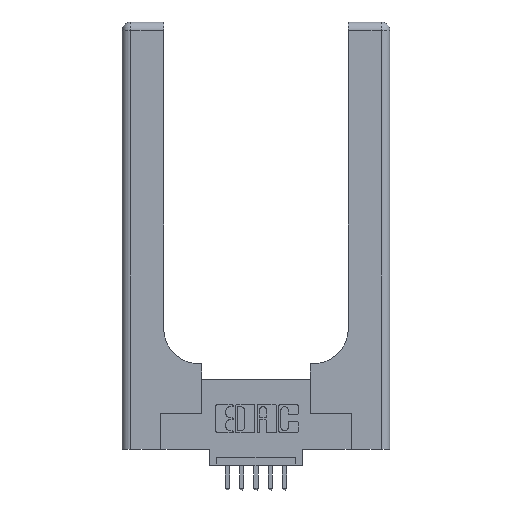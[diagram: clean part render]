
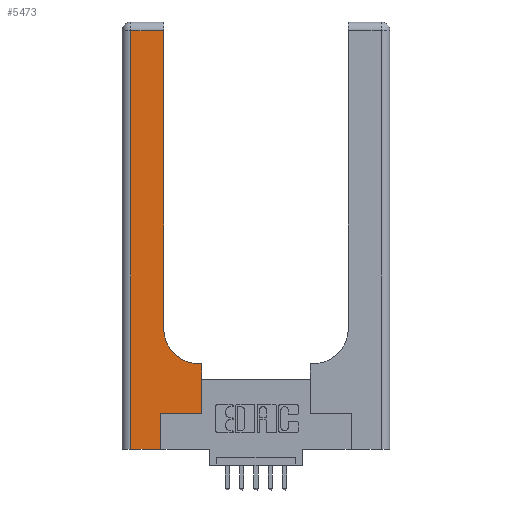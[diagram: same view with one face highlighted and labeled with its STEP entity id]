
A CAD part, top view. The second image highlights one B-rep face of the part: STEP entity #5473.
In plain terms, the highlighted planar face has unit normal (0, 0, 1).
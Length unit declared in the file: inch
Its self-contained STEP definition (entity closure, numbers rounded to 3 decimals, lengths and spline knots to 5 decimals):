
#152 = CARTESIAN_POINT ( 'NONE',  ( 0.5585, 0.25, 0.37 ) ) ;
#230 = ORIENTED_EDGE ( 'NONE', *, *, #11405, .T. ) ;
#249 = CARTESIAN_POINT ( 'NONE',  ( 0., 2.94, 0.37 ) ) ;
#283 = LINE ( 'NONE', #249, #8684 ) ;
#337 = VECTOR ( 'NONE', #8981, 39.37008 ) ;
#378 = EDGE_CURVE ( 'NONE', #619, #12434, #14074, .T. ) ;
#619 = VERTEX_POINT ( 'NONE', #13380 ) ;
#1265 = VERTEX_POINT ( 'NONE', #7395 ) ;
#1272 = VERTEX_POINT ( 'NONE', #13917 ) ;
#1301 = VECTOR ( 'NONE', #12759, 39.37008 ) ;
#1529 = CARTESIAN_POINT ( 'NONE',  ( 0.2915, 0.6, 0.37 ) ) ;
#1582 = VECTOR ( 'NONE', #13631, 39.37008 ) ;
#1648 = EDGE_CURVE ( 'NONE', #12434, #12948, #14066, .T. ) ;
#2169 = VECTOR ( 'NONE', #9839, 39.37008 ) ;
#2239 = FACE_OUTER_BOUND ( 'NONE', #4041, .T. ) ;
#2675 = CARTESIAN_POINT ( 'NONE',  ( 0.2915, 3., 0.37 ) ) ;
#3455 = CARTESIAN_POINT ( 'NONE',  ( 0.06, 3., 0.37 ) ) ;
#3541 = DIRECTION ( 'NONE',  ( -1., 0., 0. ) ) ;
#3590 = CARTESIAN_POINT ( 'NONE',  ( 0., 0., 0.37 ) ) ;
#4041 = EDGE_LOOP ( 'NONE', ( #7952, #12096, #12015, #12337, #10418, #4340, #6895, #230, #8018 ) ) ;
#4224 = VERTEX_POINT ( 'NONE', #6882 ) ;
#4260 = LINE ( 'NONE', #11627, #9775 ) ;
#4294 = DIRECTION ( 'NONE',  ( -1., 0., 0. ) ) ;
#4340 = ORIENTED_EDGE ( 'NONE', *, *, #13875, .T. ) ;
#4471 = CARTESIAN_POINT ( 'NONE',  ( 0.2915, 2.94, 0.37 ) ) ;
#4515 = CARTESIAN_POINT ( 'NONE',  ( 0.2915, 0.85, 0.37 ) ) ;
#4561 = DIRECTION ( 'NONE',  ( 0., -1., 0. ) ) ;
#4998 = DIRECTION ( 'NONE',  ( 0., 1., 0. ) ) ;
#5152 = EDGE_CURVE ( 'NONE', #4224, #9537, #7293, .T. ) ;
#5308 = CARTESIAN_POINT ( 'NONE',  ( 0., 3., 0.37 ) ) ;
#5473 = ADVANCED_FACE ( 'NONE', ( #2239 ), #9684, .F. ) ;
#5877 = EDGE_CURVE ( 'NONE', #1272, #1265, #4260, .T. ) ;
#6073 = LINE ( 'NONE', #13924, #1301 ) ;
#6106 = AXIS2_PLACEMENT_3D ( 'NONE', #7745, #11986, #8670 ) ;
#6204 = VERTEX_POINT ( 'NONE', #8912 ) ;
#6341 = AXIS2_PLACEMENT_3D ( 'NONE', #5308, #9827, #4294 ) ;
#6810 = LINE ( 'NONE', #3455, #8381 ) ;
#6859 = EDGE_CURVE ( 'NONE', #11449, #1272, #10608, .T. ) ;
#6882 = CARTESIAN_POINT ( 'NONE',  ( 0.5585, 0.25, 0.37 ) ) ;
#6895 = ORIENTED_EDGE ( 'NONE', *, *, #5152, .T. ) ;
#7106 = DIRECTION ( 'NONE',  ( 0., 1., 0. ) ) ;
#7293 = LINE ( 'NONE', #152, #2169 ) ;
#7395 = CARTESIAN_POINT ( 'NONE',  ( 0.269, 0.25, 0.37 ) ) ;
#7621 = EDGE_CURVE ( 'NONE', #6204, #11449, #6810, .T. ) ;
#7745 = CARTESIAN_POINT ( 'NONE',  ( 0.5415, 0.85, 0.37 ) ) ;
#7952 = ORIENTED_EDGE ( 'NONE', *, *, #1648, .T. ) ;
#8018 = ORIENTED_EDGE ( 'NONE', *, *, #378, .T. ) ;
#8381 = VECTOR ( 'NONE', #4561, 39.37008 ) ;
#8395 = CARTESIAN_POINT ( 'NONE',  ( 0.5585, 0.6, 0.37 ) ) ;
#8670 = DIRECTION ( 'NONE',  ( 1., 0., 0. ) ) ;
#8684 = VECTOR ( 'NONE', #3541, 39.37008 ) ;
#8912 = CARTESIAN_POINT ( 'NONE',  ( 0.06, 2.94, 0.37 ) ) ;
#8981 = DIRECTION ( 'NONE',  ( 1., 0., 0. ) ) ;
#9537 = VERTEX_POINT ( 'NONE', #8395 ) ;
#9684 = PLANE ( 'NONE',  #6341 ) ;
#9775 = VECTOR ( 'NONE', #4998, 39.37008 ) ;
#9827 = DIRECTION ( 'NONE',  ( 0., 0., -1. ) ) ;
#9839 = DIRECTION ( 'NONE',  ( 0., 1., 0. ) ) ;
#10418 = ORIENTED_EDGE ( 'NONE', *, *, #5877, .T. ) ;
#10608 = LINE ( 'NONE', #3590, #337 ) ;
#11405 = EDGE_CURVE ( 'NONE', #9537, #619, #11517, .T. ) ;
#11449 = VERTEX_POINT ( 'NONE', #11586 ) ;
#11517 = LINE ( 'NONE', #1529, #1582 ) ;
#11586 = CARTESIAN_POINT ( 'NONE',  ( 0.06, 0., 0.37 ) ) ;
#11627 = CARTESIAN_POINT ( 'NONE',  ( 0.269, 0., 0.37 ) ) ;
#11986 = DIRECTION ( 'NONE',  ( 0., 0., -1. ) ) ;
#12015 = ORIENTED_EDGE ( 'NONE', *, *, #7621, .T. ) ;
#12096 = ORIENTED_EDGE ( 'NONE', *, *, #13740, .T. ) ;
#12337 = ORIENTED_EDGE ( 'NONE', *, *, #6859, .T. ) ;
#12434 = VERTEX_POINT ( 'NONE', #4515 ) ;
#12759 = DIRECTION ( 'NONE',  ( 1., 0., 0. ) ) ;
#12948 = VERTEX_POINT ( 'NONE', #4471 ) ;
#13042 = VECTOR ( 'NONE', #7106, 39.37008 ) ;
#13380 = CARTESIAN_POINT ( 'NONE',  ( 0.5415, 0.6, 0.37 ) ) ;
#13631 = DIRECTION ( 'NONE',  ( -1., 0., 0. ) ) ;
#13740 = EDGE_CURVE ( 'NONE', #12948, #6204, #283, .T. ) ;
#13875 = EDGE_CURVE ( 'NONE', #1265, #4224, #6073, .T. ) ;
#13917 = CARTESIAN_POINT ( 'NONE',  ( 0.269, 0., 0.37 ) ) ;
#13924 = CARTESIAN_POINT ( 'NONE',  ( 0.269, 0.25, 0.37 ) ) ;
#14066 = LINE ( 'NONE', #2675, #13042 ) ;
#14074 = CIRCLE ( 'NONE', #6106, 0.25 ) ;
